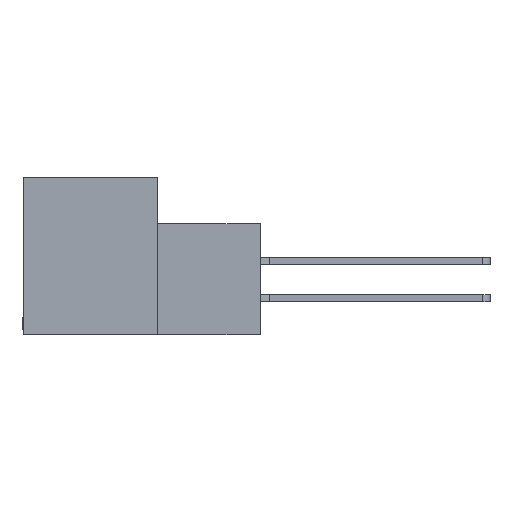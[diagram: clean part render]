
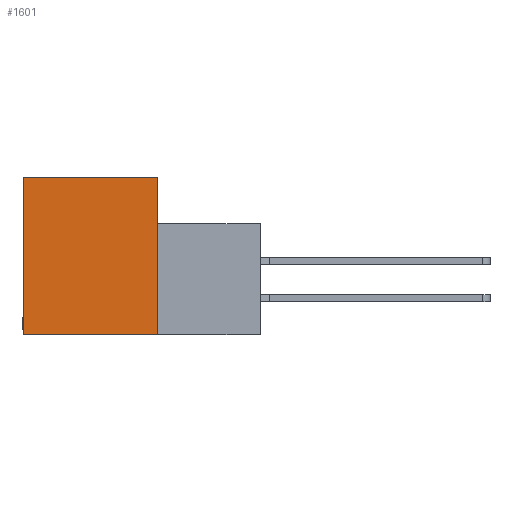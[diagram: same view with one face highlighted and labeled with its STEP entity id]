
A CAD part, left-side view. The second image highlights one B-rep face of the part: STEP entity #1601.
In plain terms, the highlighted planar face has unit normal (-1, 0, 0).
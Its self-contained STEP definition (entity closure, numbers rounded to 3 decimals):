
#1183 = VERTEX_POINT ( 'NONE', #7616 ) ;
#1272 = EDGE_CURVE ( 'NONE', #18055, #2036, #4056, .T. ) ;
#1601 = ADVANCED_FACE ( 'NONE', ( #21760 ), #23538, .F. ) ;
#2036 = VERTEX_POINT ( 'NONE', #21727 ) ;
#2589 = ORIENTED_EDGE ( 'NONE', *, *, #1272, .F. ) ;
#3068 = DIRECTION ( 'NONE',  ( 0., 0., -1. ) ) ;
#3128 = CARTESIAN_POINT ( 'NONE',  ( 0., 0., 0. ) ) ;
#3677 = CARTESIAN_POINT ( 'NONE',  ( 0., 11.506, -13.487 ) ) ;
#4056 = LINE ( 'NONE', #3677, #26693 ) ;
#4814 = CARTESIAN_POINT ( 'NONE',  ( 0., 11.506, 0. ) ) ;
#5076 = CARTESIAN_POINT ( 'NONE',  ( 0., 0., -13.487 ) ) ;
#7616 = CARTESIAN_POINT ( 'NONE',  ( 0., 0., 0. ) ) ;
#9449 = DIRECTION ( 'NONE',  ( 0., -1., 0. ) ) ;
#10741 = EDGE_CURVE ( 'NONE', #27479, #18055, #10857, .T. ) ;
#10857 = LINE ( 'NONE', #28467, #15775 ) ;
#10895 = EDGE_LOOP ( 'NONE', ( #15400, #17684, #19766, #2589 ) ) ;
#11261 = AXIS2_PLACEMENT_3D ( 'NONE', #3128, #23247, #25775 ) ;
#11445 = CARTESIAN_POINT ( 'NONE',  ( 0., 11.506, -13.487 ) ) ;
#13819 = EDGE_CURVE ( 'NONE', #2036, #1183, #16719, .T. ) ;
#15201 = DIRECTION ( 'NONE',  ( 0., 1., 0. ) ) ;
#15400 = ORIENTED_EDGE ( 'NONE', *, *, #10741, .F. ) ;
#15775 = VECTOR ( 'NONE', #15201, 1000. ) ;
#16545 = CARTESIAN_POINT ( 'NONE',  ( 0., 0., 0. ) ) ;
#16719 = LINE ( 'NONE', #4814, #19575 ) ;
#17684 = ORIENTED_EDGE ( 'NONE', *, *, #23082, .F. ) ;
#18055 = VERTEX_POINT ( 'NONE', #11445 ) ;
#19516 = DIRECTION ( 'NONE',  ( 0., 0., 1. ) ) ;
#19575 = VECTOR ( 'NONE', #9449, 1000. ) ;
#19766 = ORIENTED_EDGE ( 'NONE', *, *, #13819, .F. ) ;
#21727 = CARTESIAN_POINT ( 'NONE',  ( 0., 11.506, 0. ) ) ;
#21760 = FACE_OUTER_BOUND ( 'NONE', #10895, .T. ) ;
#23082 = EDGE_CURVE ( 'NONE', #1183, #27479, #26359, .T. ) ;
#23247 = DIRECTION ( 'NONE',  ( 1., 0., 0. ) ) ;
#23538 = PLANE ( 'NONE',  #11261 ) ;
#23541 = VECTOR ( 'NONE', #3068, 1000. ) ;
#25775 = DIRECTION ( 'NONE',  ( 0., 0., -1. ) ) ;
#26359 = LINE ( 'NONE', #16545, #23541 ) ;
#26693 = VECTOR ( 'NONE', #19516, 1000. ) ;
#27479 = VERTEX_POINT ( 'NONE', #5076 ) ;
#28467 = CARTESIAN_POINT ( 'NONE',  ( 0., -8.814, -13.487 ) ) ;
